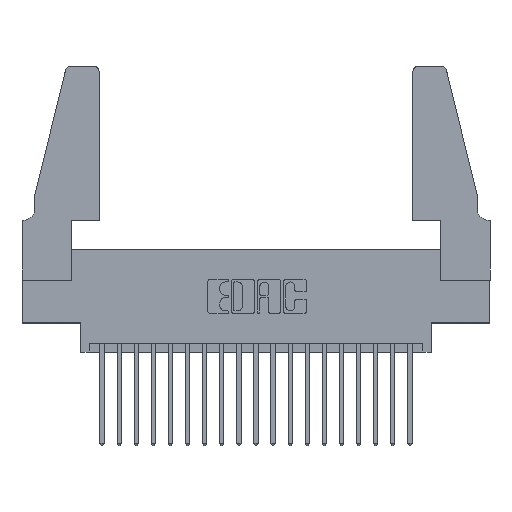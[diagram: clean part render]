
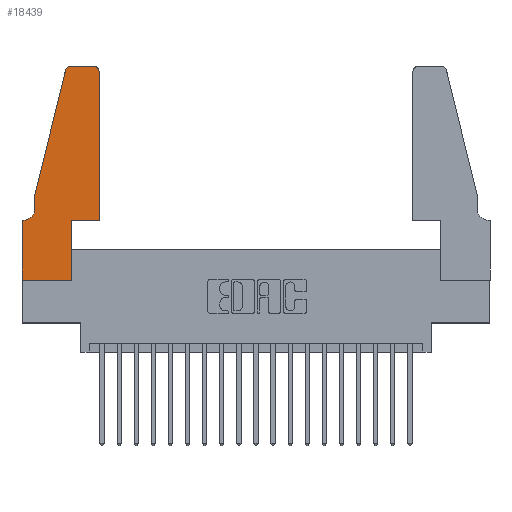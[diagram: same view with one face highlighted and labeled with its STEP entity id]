
A CAD part, top view. The second image highlights one B-rep face of the part: STEP entity #18439.
In plain terms, the highlighted planar face has unit normal (0, 0, 1).
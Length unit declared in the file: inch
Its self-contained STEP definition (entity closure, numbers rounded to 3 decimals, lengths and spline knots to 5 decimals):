
#86 = EDGE_CURVE ( 'NONE', #12670, #4691, #12402, .T. ) ;
#106 = VECTOR ( 'NONE', #12364, 39.37008 ) ;
#202 = CARTESIAN_POINT ( 'NONE',  ( 0., 0.35, 0.37 ) ) ;
#640 = EDGE_CURVE ( 'NONE', #6283, #3578, #16910, .T. ) ;
#690 = ORIENTED_EDGE ( 'NONE', *, *, #14890, .T. ) ;
#1018 = CIRCLE ( 'NONE', #14963, 0.03 ) ;
#1085 = ORIENTED_EDGE ( 'NONE', *, *, #12391, .T. ) ;
#1508 = ORIENTED_EDGE ( 'NONE', *, *, #19530, .T. ) ;
#1676 = DIRECTION ( 'NONE',  ( 0., 1., 0. ) ) ;
#1721 = CARTESIAN_POINT ( 'NONE',  ( 0., 0.35, 0.37 ) ) ;
#1898 = DIRECTION ( 'NONE',  ( 1., 0., 0. ) ) ;
#2205 = LINE ( 'NONE', #5282, #10784 ) ;
#2231 = CARTESIAN_POINT ( 'NONE',  ( 0.0055, 0.42, 0.37 ) ) ;
#2704 = LINE ( 'NONE', #16744, #6575 ) ;
#2729 = ORIENTED_EDGE ( 'NONE', *, *, #640, .T. ) ;
#3204 = VERTEX_POINT ( 'NONE', #19722 ) ;
#3288 = DIRECTION ( 'NONE',  ( 1., 0., 0. ) ) ;
#3501 = CARTESIAN_POINT ( 'NONE',  ( 0.25487, 1.22718, 0.37 ) ) ;
#3571 = ORIENTED_EDGE ( 'NONE', *, *, #5391, .T. ) ;
#3578 = VERTEX_POINT ( 'NONE', #202 ) ;
#3955 = DIRECTION ( 'NONE',  ( -1., 0., 0. ) ) ;
#3972 = LINE ( 'NONE', #9718, #19410 ) ;
#4003 = ORIENTED_EDGE ( 'NONE', *, *, #5955, .T. ) ;
#4100 = ORIENTED_EDGE ( 'NONE', *, *, #7207, .T. ) ;
#4277 = VERTEX_POINT ( 'NONE', #14550 ) ;
#4611 = LINE ( 'NONE', #16953, #5639 ) ;
#4614 = CARTESIAN_POINT ( 'NONE',  ( 0.4505, 0.35, 0.37 ) ) ;
#4664 = CARTESIAN_POINT ( 'NONE',  ( 0.0055, 0.35, 0.37 ) ) ;
#4691 = VERTEX_POINT ( 'NONE', #4614 ) ;
#5010 = DIRECTION ( 'NONE',  ( -1., 0., 0. ) ) ;
#5097 = DIRECTION ( 'NONE',  ( 0., 0., 1. ) ) ;
#5267 = DIRECTION ( 'NONE',  ( 0., 1., 0. ) ) ;
#5282 = CARTESIAN_POINT ( 'NONE',  ( 0., 0., 0.37 ) ) ;
#5359 = ORIENTED_EDGE ( 'NONE', *, *, #10315, .T. ) ;
#5391 = EDGE_CURVE ( 'NONE', #17009, #18453, #10495, .T. ) ;
#5639 = VECTOR ( 'NONE', #7753, 39.37008 ) ;
#5760 = CARTESIAN_POINT ( 'NONE',  ( 0.0755, 0.35, 0.37 ) ) ;
#5815 = CARTESIAN_POINT ( 'NONE',  ( 0.284, 1.25, 0.37 ) ) ;
#5955 = EDGE_CURVE ( 'NONE', #3204, #6283, #9470, .T. ) ;
#6065 = VERTEX_POINT ( 'NONE', #13581 ) ;
#6283 = VERTEX_POINT ( 'NONE', #4664 ) ;
#6394 = DIRECTION ( 'NONE',  ( 0., 0., 1. ) ) ;
#6575 = VECTOR ( 'NONE', #7529, 39.37008 ) ;
#7084 = DIRECTION ( 'NONE',  ( -1., 0., 0. ) ) ;
#7207 = EDGE_CURVE ( 'NONE', #18264, #17009, #15457, .T. ) ;
#7529 = DIRECTION ( 'NONE',  ( 0., -1., 0. ) ) ;
#7548 = EDGE_CURVE ( 'NONE', #6065, #18264, #1018, .T. ) ;
#7753 = DIRECTION ( 'NONE',  ( 0., -1., 0. ) ) ;
#8198 = PLANE ( 'NONE',  #12150 ) ;
#8475 = ORIENTED_EDGE ( 'NONE', *, *, #86, .T. ) ;
#8814 = VERTEX_POINT ( 'NONE', #16225 ) ;
#8869 = VERTEX_POINT ( 'NONE', #10250 ) ;
#8980 = CARTESIAN_POINT ( 'NONE',  ( 0.284, 1.22, 0.37 ) ) ;
#9470 = CIRCLE ( 'NONE', #18804, 0.07 ) ;
#9718 = CARTESIAN_POINT ( 'NONE',  ( 0.4505, 0.35, 0.37 ) ) ;
#10081 = ORIENTED_EDGE ( 'NONE', *, *, #13247, .T. ) ;
#10250 = CARTESIAN_POINT ( 'NONE',  ( 0., 0., 0.37 ) ) ;
#10270 = ORIENTED_EDGE ( 'NONE', *, *, #14771, .T. ) ;
#10315 = EDGE_CURVE ( 'NONE', #18453, #4277, #12470, .T. ) ;
#10430 = LINE ( 'NONE', #16177, #13559 ) ;
#10495 = CIRCLE ( 'NONE', #18756, 0.03 ) ;
#10567 = DIRECTION ( 'NONE',  ( 1., 0., 0. ) ) ;
#10784 = VECTOR ( 'NONE', #1898, 39.37008 ) ;
#10885 = CARTESIAN_POINT ( 'NONE',  ( 0.4205, 1.25, 0.37 ) ) ;
#11287 = CARTESIAN_POINT ( 'NONE',  ( 0.4505, 0.35, 0.37 ) ) ;
#11867 = VECTOR ( 'NONE', #7084, 39.37008 ) ;
#11930 = VECTOR ( 'NONE', #3288, 39.37008 ) ;
#12150 = AXIS2_PLACEMENT_3D ( 'NONE', #1721, #5097, #15963 ) ;
#12364 = DIRECTION ( 'NONE',  ( -0.239, -0.971, 0. ) ) ;
#12391 = EDGE_CURVE ( 'NONE', #8869, #8814, #2205, .T. ) ;
#12402 = LINE ( 'NONE', #11287, #11930 ) ;
#12470 = LINE ( 'NONE', #16885, #106 ) ;
#12482 = ORIENTED_EDGE ( 'NONE', *, *, #7548, .T. ) ;
#12670 = VERTEX_POINT ( 'NONE', #18491 ) ;
#13240 = FACE_OUTER_BOUND ( 'NONE', #18767, .T. ) ;
#13247 = EDGE_CURVE ( 'NONE', #4277, #3204, #2704, .T. ) ;
#13338 = CARTESIAN_POINT ( 'NONE',  ( 0.2605, 1.25, 0.37 ) ) ;
#13373 = DIRECTION ( 'NONE',  ( 0., 0., -1. ) ) ;
#13559 = VECTOR ( 'NONE', #5267, 39.37008 ) ;
#13581 = CARTESIAN_POINT ( 'NONE',  ( 0.4505, 1.22, 0.37 ) ) ;
#14550 = CARTESIAN_POINT ( 'NONE',  ( 0.0755, 0.5, 0.37 ) ) ;
#14771 = EDGE_CURVE ( 'NONE', #4691, #6065, #3972, .T. ) ;
#14890 = EDGE_CURVE ( 'NONE', #8814, #12670, #10430, .T. ) ;
#14963 = AXIS2_PLACEMENT_3D ( 'NONE', #15653, #6394, #17161 ) ;
#15457 = LINE ( 'NONE', #13338, #11867 ) ;
#15653 = CARTESIAN_POINT ( 'NONE',  ( 0.4205, 1.22, 0.37 ) ) ;
#15963 = DIRECTION ( 'NONE',  ( 1., 0., 0. ) ) ;
#16177 = CARTESIAN_POINT ( 'NONE',  ( 0.2865, 0.35, 0.37 ) ) ;
#16225 = CARTESIAN_POINT ( 'NONE',  ( 0.2865, 0., 0.37 ) ) ;
#16744 = CARTESIAN_POINT ( 'NONE',  ( 0.0755, 0.5, 0.37 ) ) ;
#16885 = CARTESIAN_POINT ( 'NONE',  ( 0.0755, 0.5, 0.37 ) ) ;
#16910 = LINE ( 'NONE', #5760, #19451 ) ;
#16953 = CARTESIAN_POINT ( 'NONE',  ( 0., 0., 0.37 ) ) ;
#17009 = VERTEX_POINT ( 'NONE', #5815 ) ;
#17161 = DIRECTION ( 'NONE',  ( 1., 0., 0. ) ) ;
#18264 = VERTEX_POINT ( 'NONE', #10885 ) ;
#18439 = ADVANCED_FACE ( 'NONE', ( #13240 ), #8198, .T. ) ;
#18453 = VERTEX_POINT ( 'NONE', #3501 ) ;
#18491 = CARTESIAN_POINT ( 'NONE',  ( 0.2865, 0.35, 0.37 ) ) ;
#18756 = AXIS2_PLACEMENT_3D ( 'NONE', #8980, #19610, #10567 ) ;
#18767 = EDGE_LOOP ( 'NONE', ( #4100, #3571, #5359, #10081, #4003, #2729, #1508, #1085, #690, #8475, #10270, #12482 ) ) ;
#18804 = AXIS2_PLACEMENT_3D ( 'NONE', #2231, #13373, #3955 ) ;
#19410 = VECTOR ( 'NONE', #1676, 39.37008 ) ;
#19451 = VECTOR ( 'NONE', #5010, 39.37008 ) ;
#19530 = EDGE_CURVE ( 'NONE', #3578, #8869, #4611, .T. ) ;
#19610 = DIRECTION ( 'NONE',  ( 0., 0., 1. ) ) ;
#19722 = CARTESIAN_POINT ( 'NONE',  ( 0.0755, 0.42, 0.37 ) ) ;
